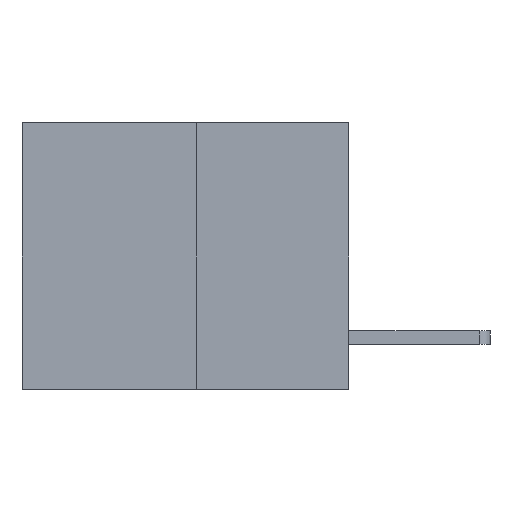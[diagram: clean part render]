
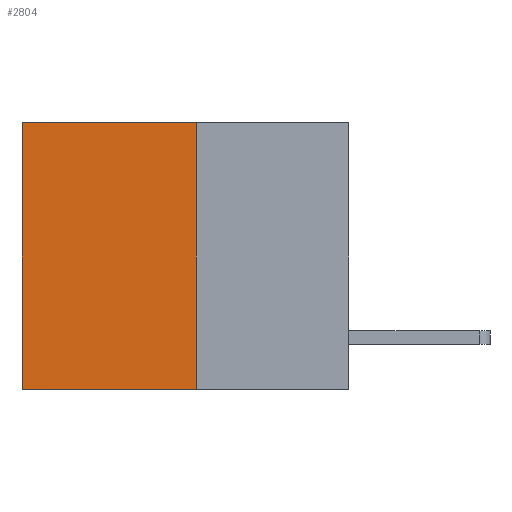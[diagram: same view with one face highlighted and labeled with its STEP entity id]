
A CAD part, left-side view. The second image highlights one B-rep face of the part: STEP entity #2804.
In plain terms, the highlighted planar face has unit normal (-1, 0, 0).
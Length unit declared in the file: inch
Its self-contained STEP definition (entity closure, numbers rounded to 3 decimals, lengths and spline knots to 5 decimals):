
#24 = ORIENTED_EDGE ( 'NONE', *, *, #1498, .T. ) ;
#877 = CARTESIAN_POINT ( 'NONE',  ( 0.3165, 0.28, -0.49 ) ) ;
#960 = VERTEX_POINT ( 'NONE', #4744 ) ;
#1484 = AXIS2_PLACEMENT_3D ( 'NONE', #3060, #6198, #2376 ) ;
#1498 = EDGE_CURVE ( 'NONE', #7535, #2767, #6348, .T. ) ;
#1576 = VECTOR ( 'NONE', #5562, 39.37008 ) ;
#1627 = CARTESIAN_POINT ( 'NONE',  ( 0.3165, 0.28, -0.49 ) ) ;
#1741 = PLANE ( 'NONE',  #1484 ) ;
#2376 = DIRECTION ( 'NONE',  ( 0., 0., -1. ) ) ;
#2560 = LINE ( 'NONE', #877, #4045 ) ;
#2668 = EDGE_CURVE ( 'NONE', #2767, #960, #5610, .T. ) ;
#2755 = DIRECTION ( 'NONE',  ( 0., 0., -1. ) ) ;
#2767 = VERTEX_POINT ( 'NONE', #6817 ) ;
#2804 = ADVANCED_FACE ( 'NONE', ( #6224 ), #1741, .F. ) ;
#3060 = CARTESIAN_POINT ( 'NONE',  ( 0.3165, 0.28, -0.49 ) ) ;
#3785 = ORIENTED_EDGE ( 'NONE', *, *, #7427, .F. ) ;
#3806 = VECTOR ( 'NONE', #4606, 39.37008 ) ;
#3840 = EDGE_CURVE ( 'NONE', #5946, #960, #7204, .T. ) ;
#4045 = VECTOR ( 'NONE', #5947, 39.37008 ) ;
#4061 = EDGE_LOOP ( 'NONE', ( #6381, #4778, #3785, #24 ) ) ;
#4117 = CARTESIAN_POINT ( 'NONE',  ( 0.3165, 0.28, 0. ) ) ;
#4606 = DIRECTION ( 'NONE',  ( 0., 1., 0. ) ) ;
#4744 = CARTESIAN_POINT ( 'NONE',  ( 0.3165, 0.6, -0.49 ) ) ;
#4778 = ORIENTED_EDGE ( 'NONE', *, *, #3840, .F. ) ;
#4797 = CARTESIAN_POINT ( 'NONE',  ( 0.3165, 0.28, 0. ) ) ;
#5562 = DIRECTION ( 'NONE',  ( 0., 1., 0. ) ) ;
#5610 = LINE ( 'NONE', #5820, #5931 ) ;
#5820 = CARTESIAN_POINT ( 'NONE',  ( 0.3165, 0.6, -0.49 ) ) ;
#5931 = VECTOR ( 'NONE', #2755, 39.37008 ) ;
#5946 = VERTEX_POINT ( 'NONE', #1627 ) ;
#5947 = DIRECTION ( 'NONE',  ( 0., 0., -1. ) ) ;
#6198 = DIRECTION ( 'NONE',  ( 1., 0., 0. ) ) ;
#6224 = FACE_OUTER_BOUND ( 'NONE', #4061, .T. ) ;
#6348 = LINE ( 'NONE', #4797, #1576 ) ;
#6381 = ORIENTED_EDGE ( 'NONE', *, *, #2668, .T. ) ;
#6427 = CARTESIAN_POINT ( 'NONE',  ( 0.3165, 0.28, -0.49 ) ) ;
#6817 = CARTESIAN_POINT ( 'NONE',  ( 0.3165, 0.6, 0. ) ) ;
#7204 = LINE ( 'NONE', #6427, #3806 ) ;
#7427 = EDGE_CURVE ( 'NONE', #7535, #5946, #2560, .T. ) ;
#7535 = VERTEX_POINT ( 'NONE', #4117 ) ;
